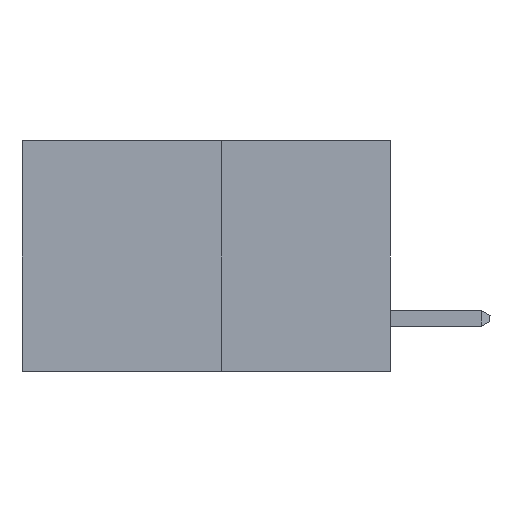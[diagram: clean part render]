
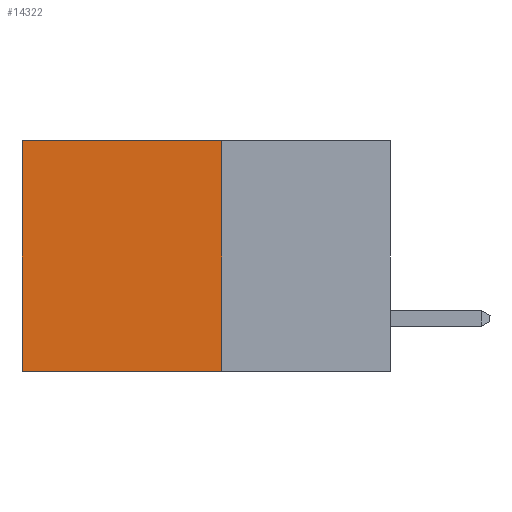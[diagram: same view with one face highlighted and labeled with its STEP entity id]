
A CAD part, left-side view. The second image highlights one B-rep face of the part: STEP entity #14322.
In plain terms, the highlighted planar face has unit normal (-1, 0, 0).
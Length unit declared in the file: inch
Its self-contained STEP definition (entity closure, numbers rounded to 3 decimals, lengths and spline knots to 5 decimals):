
#226 = CARTESIAN_POINT ( 'NONE',  ( 0.277, 0.27, -0.37 ) ) ;
#825 = VERTEX_POINT ( 'NONE', #6558 ) ;
#988 = CARTESIAN_POINT ( 'NONE',  ( 0.277, 0.27, 0. ) ) ;
#1218 = VERTEX_POINT ( 'NONE', #1993 ) ;
#1993 = CARTESIAN_POINT ( 'NONE',  ( 0.277, 0.59, -0.37 ) ) ;
#2168 = ORIENTED_EDGE ( 'NONE', *, *, #7324, .F. ) ;
#2360 = ORIENTED_EDGE ( 'NONE', *, *, #13263, .T. ) ;
#2573 = CARTESIAN_POINT ( 'NONE',  ( 0.277, 0.59, -0.37 ) ) ;
#3378 = CARTESIAN_POINT ( 'NONE',  ( 0.277, 0.27, -0.37 ) ) ;
#4004 = VECTOR ( 'NONE', #12667, 39.37008 ) ;
#4167 = ORIENTED_EDGE ( 'NONE', *, *, #8684, .T. ) ;
#4262 = FACE_OUTER_BOUND ( 'NONE', #5060, .T. ) ;
#4559 = ORIENTED_EDGE ( 'NONE', *, *, #7065, .F. ) ;
#5060 = EDGE_LOOP ( 'NONE', ( #2360, #4559, #2168, #4167 ) ) ;
#5148 = PLANE ( 'NONE',  #5214 ) ;
#5214 = AXIS2_PLACEMENT_3D ( 'NONE', #12731, #13798, #7438 ) ;
#5388 = LINE ( 'NONE', #8673, #13662 ) ;
#6558 = CARTESIAN_POINT ( 'NONE',  ( 0.277, 0.59, 0. ) ) ;
#6825 = VECTOR ( 'NONE', #11496, 39.37008 ) ;
#7065 = EDGE_CURVE ( 'NONE', #8197, #1218, #10010, .T. ) ;
#7113 = DIRECTION ( 'NONE',  ( 0., 0., -1. ) ) ;
#7324 = EDGE_CURVE ( 'NONE', #13635, #8197, #9488, .T. ) ;
#7438 = DIRECTION ( 'NONE',  ( 0., 0., -1. ) ) ;
#8197 = VERTEX_POINT ( 'NONE', #3378 ) ;
#8673 = CARTESIAN_POINT ( 'NONE',  ( 0.277, 0.27, 0. ) ) ;
#8684 = EDGE_CURVE ( 'NONE', #13635, #825, #5388, .T. ) ;
#8934 = DIRECTION ( 'NONE',  ( 0., 1., 0. ) ) ;
#9157 = CARTESIAN_POINT ( 'NONE',  ( 0.277, 0.27, -0.37 ) ) ;
#9488 = LINE ( 'NONE', #9157, #12242 ) ;
#10010 = LINE ( 'NONE', #226, #4004 ) ;
#11496 = DIRECTION ( 'NONE',  ( 0., 0., -1. ) ) ;
#12242 = VECTOR ( 'NONE', #7113, 39.37008 ) ;
#12511 = LINE ( 'NONE', #2573, #6825 ) ;
#12667 = DIRECTION ( 'NONE',  ( 0., 1., 0. ) ) ;
#12731 = CARTESIAN_POINT ( 'NONE',  ( 0.277, 0.27, -0.37 ) ) ;
#13263 = EDGE_CURVE ( 'NONE', #825, #1218, #12511, .T. ) ;
#13635 = VERTEX_POINT ( 'NONE', #988 ) ;
#13662 = VECTOR ( 'NONE', #8934, 39.37008 ) ;
#13798 = DIRECTION ( 'NONE',  ( 1., 0., 0. ) ) ;
#14322 = ADVANCED_FACE ( 'NONE', ( #4262 ), #5148, .F. ) ;
